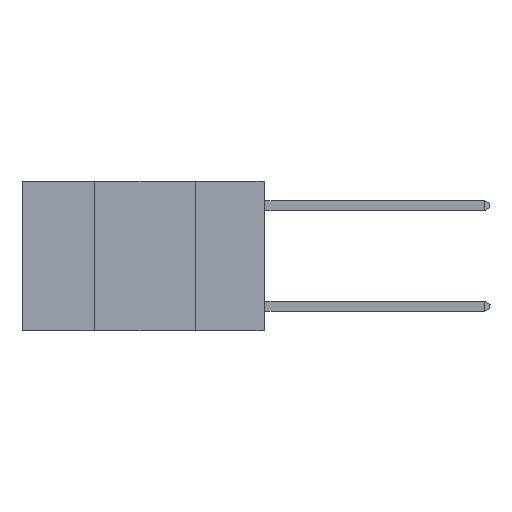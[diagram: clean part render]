
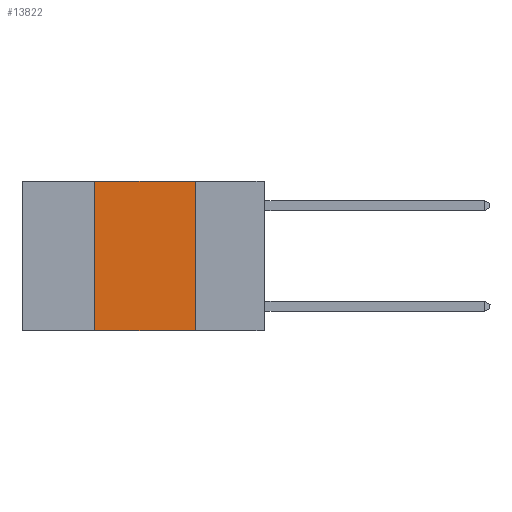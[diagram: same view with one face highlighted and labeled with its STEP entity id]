
A CAD part, left-side view. The second image highlights one B-rep face of the part: STEP entity #13822.
In plain terms, the highlighted planar face has unit normal (-1, 0, 0).
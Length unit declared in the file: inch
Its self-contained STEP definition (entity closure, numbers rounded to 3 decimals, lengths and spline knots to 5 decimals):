
#789 = DIRECTION ( 'NONE',  ( 0., 0., -1. ) ) ;
#988 = VECTOR ( 'NONE', #5549, 39.37008 ) ;
#1096 = CARTESIAN_POINT ( 'NONE',  ( 0., 0.6, -0.37 ) ) ;
#1566 = CARTESIAN_POINT ( 'NONE',  ( 0., 0.6, 0. ) ) ;
#2329 = LINE ( 'NONE', #11030, #5312 ) ;
#2572 = EDGE_CURVE ( 'NONE', #14210, #3903, #16066, .T. ) ;
#2745 = DIRECTION ( 'NONE',  ( 0., -1., 0. ) ) ;
#2835 = DIRECTION ( 'NONE',  ( 0., -1., 0. ) ) ;
#3281 = CARTESIAN_POINT ( 'NONE',  ( 0., 0.17, -0.37 ) ) ;
#3316 = CARTESIAN_POINT ( 'NONE',  ( 0., 0.6, 0. ) ) ;
#3903 = VERTEX_POINT ( 'NONE', #3281 ) ;
#4263 = CARTESIAN_POINT ( 'NONE',  ( 0., 0.17, 0. ) ) ;
#4325 = VERTEX_POINT ( 'NONE', #6522 ) ;
#4460 = EDGE_CURVE ( 'NONE', #9511, #3903, #10669, .T. ) ;
#5308 = AXIS2_PLACEMENT_3D ( 'NONE', #3316, #8414, #789 ) ;
#5312 = VECTOR ( 'NONE', #12258, 39.37008 ) ;
#5549 = DIRECTION ( 'NONE',  ( 0., 0., -1. ) ) ;
#5729 = EDGE_CURVE ( 'NONE', #4325, #9511, #8868, .T. ) ;
#6382 = FACE_OUTER_BOUND ( 'NONE', #9421, .T. ) ;
#6522 = CARTESIAN_POINT ( 'NONE',  ( 0., 0.42, 0. ) ) ;
#7130 = PLANE ( 'NONE',  #5308 ) ;
#8414 = DIRECTION ( 'NONE',  ( 1., 0., 0. ) ) ;
#8471 = CARTESIAN_POINT ( 'NONE',  ( 0., 0.17, 0. ) ) ;
#8860 = ORIENTED_EDGE ( 'NONE', *, *, #4460, .F. ) ;
#8868 = LINE ( 'NONE', #1566, #12140 ) ;
#8887 = ORIENTED_EDGE ( 'NONE', *, *, #5729, .F. ) ;
#9062 = ORIENTED_EDGE ( 'NONE', *, *, #11203, .F. ) ;
#9421 = EDGE_LOOP ( 'NONE', ( #8860, #8887, #9062, #9783 ) ) ;
#9511 = VERTEX_POINT ( 'NONE', #8471 ) ;
#9783 = ORIENTED_EDGE ( 'NONE', *, *, #2572, .T. ) ;
#10669 = LINE ( 'NONE', #4263, #988 ) ;
#11030 = CARTESIAN_POINT ( 'NONE',  ( 0., 0.42, 0. ) ) ;
#11203 = EDGE_CURVE ( 'NONE', #14210, #4325, #2329, .T. ) ;
#11514 = CARTESIAN_POINT ( 'NONE',  ( 0., 0.42, -0.37 ) ) ;
#12140 = VECTOR ( 'NONE', #2835, 39.37008 ) ;
#12258 = DIRECTION ( 'NONE',  ( 0., 0., 1. ) ) ;
#12816 = VECTOR ( 'NONE', #2745, 39.37008 ) ;
#13822 = ADVANCED_FACE ( 'NONE', ( #6382 ), #7130, .F. ) ;
#14210 = VERTEX_POINT ( 'NONE', #11514 ) ;
#16066 = LINE ( 'NONE', #1096, #12816 ) ;
